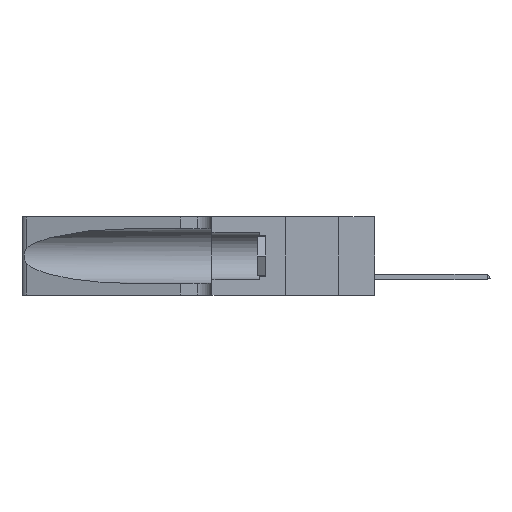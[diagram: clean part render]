
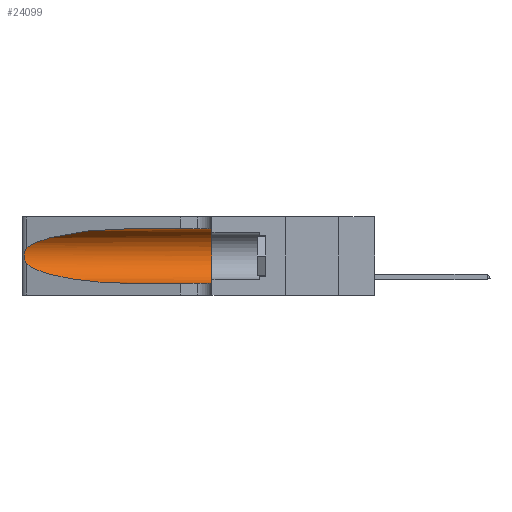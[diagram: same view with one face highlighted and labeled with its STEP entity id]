
A CAD part, left-side view. The second image highlights one B-rep face of the part: STEP entity #24099.
In plain terms, the highlighted cylindrical face has radius 3.308 mm (diameter 6.617 mm), a partial arc.
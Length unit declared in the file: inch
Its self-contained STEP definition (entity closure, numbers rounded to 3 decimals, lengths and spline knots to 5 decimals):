
#1803 = CARTESIAN_POINT ( 'NONE',  ( 0.18966, 0.96281, 0.31525 ) ) ;
#2038 = VERTEX_POINT ( 'NONE', #26045 ) ;
#2220 =( BOUNDED_CURVE ( )  B_SPLINE_CURVE ( 3, ( #16921, #1803, #21781, #4312 ),
 .UNSPECIFIED., .F., .F. ) 
 B_SPLINE_CURVE_WITH_KNOTS ( ( 4, 4 ),
 ( 1.5708, 2.84003 ),
 .UNSPECIFIED. ) 
 CURVE ( )  GEOMETRIC_REPRESENTATION_ITEM ( )  RATIONAL_B_SPLINE_CURVE ( ( 1., 0.87, 0.87, 1. ) ) 
 REPRESENTATION_ITEM ( '' )  );
#2319 = CARTESIAN_POINT ( 'NONE',  ( 0.25639, 1.23184, 0.21858 ) ) ;
#2524 = ORIENTED_EDGE ( 'NONE', *, *, #21922, .F. ) ;
#2647 = AXIS2_PLACEMENT_3D ( 'NONE', #31741, #8667, #11058 ) ;
#4072 = CARTESIAN_POINT ( 'NONE',  ( 0.1305, 0.35, 0.185 ) ) ;
#4312 = CARTESIAN_POINT ( 'NONE',  ( 0.25487, 1.22718, 0.22369 ) ) ;
#4384 = ORIENTED_EDGE ( 'NONE', *, *, #21764, .F. ) ;
#4485 = AXIS2_PLACEMENT_3D ( 'NONE', #4072, #21757, #11711 ) ;
#4623 = CARTESIAN_POINT ( 'NONE',  ( 0.26075, 1.23896, 0.19203 ) ) ;
#4813 = CARTESIAN_POINT ( 'NONE',  ( 0.25487, 1.22718, 0.22369 ) ) ;
#5014 = B_SPLINE_CURVE_WITH_KNOTS ( 'NONE', 3,
 ( #4813, #27294, #2319, #9725, #14914, #7183, #4623, #20005, #9912, #27611, #7294, #7500, #7412, #25134 ),
 .UNSPECIFIED., .F., .F.,
 ( 4, 2, 2, 2, 2, 2, 4 ),
 ( 0., 0.00027, 0.00053, 0.00107, 0.0016, 0.00187, 0.00214 ),
 .UNSPECIFIED. ) ;
#5573 = FACE_OUTER_BOUND ( 'NONE', #24250, .T. ) ;
#6628 = CARTESIAN_POINT ( 'NONE',  ( 0.1305, 0.72297, 0.31525 ) ) ;
#7183 = CARTESIAN_POINT ( 'NONE',  ( 0.26018, 1.23835, 0.19895 ) ) ;
#7256 = CARTESIAN_POINT ( 'NONE',  ( 0.1305, 0.72297, 0.05475 ) ) ;
#7294 = CARTESIAN_POINT ( 'NONE',  ( 0.25789, 1.23486, 0.15765 ) ) ;
#7412 = CARTESIAN_POINT ( 'NONE',  ( 0.25555, 1.22993, 0.14849 ) ) ;
#7500 = CARTESIAN_POINT ( 'NONE',  ( 0.25639, 1.23186, 0.15144 ) ) ;
#7572 = CARTESIAN_POINT ( 'NONE',  ( 0.18966, 0.96281, 0.05475 ) ) ;
#7821 = ORIENTED_EDGE ( 'NONE', *, *, #13451, .T. ) ;
#8013 = CYLINDRICAL_SURFACE ( 'NONE', #2647, 0.13025 ) ;
#8667 = DIRECTION ( 'NONE',  ( 0., -1., 0. ) ) ;
#8930 = CARTESIAN_POINT ( 'NONE',  ( 0.25487, 1.22718, 0.14631 ) ) ;
#9725 = CARTESIAN_POINT ( 'NONE',  ( 0.25787, 1.23484, 0.2124 ) ) ;
#9801 = LINE ( 'NONE', #12389, #14951 ) ;
#9912 = CARTESIAN_POINT ( 'NONE',  ( 0.26017, 1.23833, 0.17102 ) ) ;
#10791 = ORIENTED_EDGE ( 'NONE', *, *, #14371, .T. ) ;
#11058 = DIRECTION ( 'NONE',  ( 0., 0., -1. ) ) ;
#11299 = LINE ( 'NONE', #12907, #12864 ) ;
#11711 = DIRECTION ( 'NONE',  ( 0., 0., 1. ) ) ;
#12281 = CARTESIAN_POINT ( 'NONE',  ( 0.1305, 0.35, 0.31525 ) ) ;
#12289 = DIRECTION ( 'NONE',  ( 0., -1., 0. ) ) ;
#12376 = EDGE_CURVE ( 'NONE', #32122, #18310, #2220, .T. ) ;
#12389 = CARTESIAN_POINT ( 'NONE',  ( 0.1305, 1.61858, 0.31525 ) ) ;
#12864 = VECTOR ( 'NONE', #18740, 39.37008 ) ;
#12907 = CARTESIAN_POINT ( 'NONE',  ( 0.1305, 1.61858, 0.05475 ) ) ;
#13331 =( BOUNDED_CURVE ( )  B_SPLINE_CURVE ( 3, ( #19859, #25104, #7572, #7256 ),
 .UNSPECIFIED., .F., .T. ) 
 B_SPLINE_CURVE_WITH_KNOTS ( ( 4, 4 ),
 ( 3.44316, 4.71239 ),
 .UNSPECIFIED. ) 
 CURVE ( )  GEOMETRIC_REPRESENTATION_ITEM ( )  RATIONAL_B_SPLINE_CURVE ( ( 1., 0.87, 0.87, 1. ) ) 
 REPRESENTATION_ITEM ( '' )  );
#13451 = EDGE_CURVE ( 'NONE', #30767, #2038, #11299, .T. ) ;
#14371 = EDGE_CURVE ( 'NONE', #22808, #30767, #13331, .T. ) ;
#14914 = CARTESIAN_POINT ( 'NONE',  ( 0.25854, 1.2359, 0.20912 ) ) ;
#14951 = VECTOR ( 'NONE', #12289, 39.37008 ) ;
#16921 = CARTESIAN_POINT ( 'NONE',  ( 0.1305, 0.72297, 0.31525 ) ) ;
#18310 = VERTEX_POINT ( 'NONE', #19786 ) ;
#18325 = EDGE_CURVE ( 'NONE', #18310, #22808, #5014, .T. ) ;
#18740 = DIRECTION ( 'NONE',  ( 0., -1., 0. ) ) ;
#19786 = CARTESIAN_POINT ( 'NONE',  ( 0.25487, 1.22718, 0.22369 ) ) ;
#19859 = CARTESIAN_POINT ( 'NONE',  ( 0.25487, 1.22718, 0.14631 ) ) ;
#20005 = CARTESIAN_POINT ( 'NONE',  ( 0.26075, 1.23896, 0.178 ) ) ;
#20336 = VERTEX_POINT ( 'NONE', #12281 ) ;
#21757 = DIRECTION ( 'NONE',  ( 0., 1., 0. ) ) ;
#21764 = EDGE_CURVE ( 'NONE', #20336, #2038, #22455, .T. ) ;
#21781 = CARTESIAN_POINT ( 'NONE',  ( 0.2373, 1.15595, 0.28018 ) ) ;
#21922 = EDGE_CURVE ( 'NONE', #32122, #20336, #9801, .T. ) ;
#22455 = CIRCLE ( 'NONE', #4485, 0.13025 ) ;
#22808 = VERTEX_POINT ( 'NONE', #8930 ) ;
#24099 = ADVANCED_FACE ( 'NONE', ( #5573 ), #8013, .F. ) ;
#24250 = EDGE_LOOP ( 'NONE', ( #28056, #27709, #10791, #7821, #4384, #2524 ) ) ;
#25104 = CARTESIAN_POINT ( 'NONE',  ( 0.2373, 1.15595, 0.08982 ) ) ;
#25134 = CARTESIAN_POINT ( 'NONE',  ( 0.25487, 1.22718, 0.14631 ) ) ;
#26045 = CARTESIAN_POINT ( 'NONE',  ( 0.1305, 0.35, 0.05475 ) ) ;
#27294 = CARTESIAN_POINT ( 'NONE',  ( 0.25555, 1.22994, 0.2215 ) ) ;
#27611 = CARTESIAN_POINT ( 'NONE',  ( 0.25856, 1.23593, 0.16098 ) ) ;
#27709 = ORIENTED_EDGE ( 'NONE', *, *, #18325, .T. ) ;
#28056 = ORIENTED_EDGE ( 'NONE', *, *, #12376, .T. ) ;
#30524 = CARTESIAN_POINT ( 'NONE',  ( 0.1305, 0.72297, 0.05475 ) ) ;
#30767 = VERTEX_POINT ( 'NONE', #30524 ) ;
#31741 = CARTESIAN_POINT ( 'NONE',  ( 0.1305, 1.61858, 0.185 ) ) ;
#32122 = VERTEX_POINT ( 'NONE', #6628 ) ;
